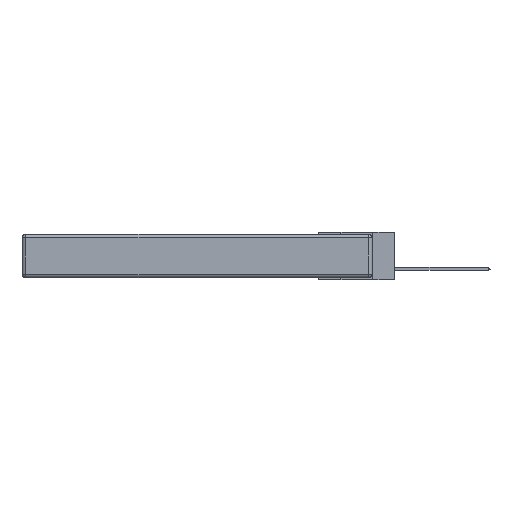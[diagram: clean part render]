
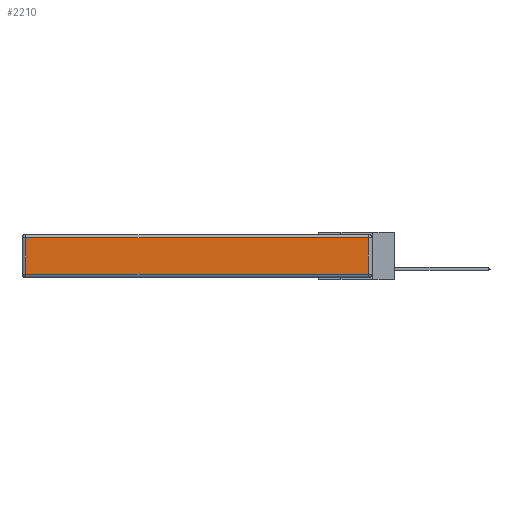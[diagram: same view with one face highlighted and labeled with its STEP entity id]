
A CAD part, left-side view. The second image highlights one B-rep face of the part: STEP entity #2210.
In plain terms, the highlighted planar face has unit normal (-1, 0, 0).
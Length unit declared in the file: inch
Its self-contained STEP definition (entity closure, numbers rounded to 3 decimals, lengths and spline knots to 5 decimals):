
#1325 = FACE_OUTER_BOUND ( 'NONE', #23199, .T. ) ;
#1782 = CARTESIAN_POINT ( 'NONE',  ( 0., 2.72, -0.343 ) ) ;
#2210 = ADVANCED_FACE ( 'NONE', ( #1325 ), #20587, .T. ) ;
#2214 = DIRECTION ( 'NONE',  ( 0., 0., 1. ) ) ;
#4475 = VECTOR ( 'NONE', #23477, 39.37008 ) ;
#6830 = CARTESIAN_POINT ( 'NONE',  ( 0., 0.03, -0.343 ) ) ;
#8288 = ORIENTED_EDGE ( 'NONE', *, *, #9230, .T. ) ;
#8354 = ORIENTED_EDGE ( 'NONE', *, *, #14554, .T. ) ;
#8678 = DIRECTION ( 'NONE',  ( 0., 0., 1. ) ) ;
#8729 = VECTOR ( 'NONE', #8678, 39.37008 ) ;
#9230 = EDGE_CURVE ( 'NONE', #17596, #16946, #21676, .T. ) ;
#9329 = LINE ( 'NONE', #11516, #4475 ) ;
#9456 = VERTEX_POINT ( 'NONE', #12620 ) ;
#10346 = DIRECTION ( 'NONE',  ( 0., 1., 0. ) ) ;
#10718 = EDGE_CURVE ( 'NONE', #9456, #15543, #23298, .T. ) ;
#11516 = CARTESIAN_POINT ( 'NONE',  ( 0., 0., -0.313 ) ) ;
#12620 = CARTESIAN_POINT ( 'NONE',  ( 0., 0.03, -0.313 ) ) ;
#12637 = CARTESIAN_POINT ( 'NONE',  ( 0., 0.03, -0.03 ) ) ;
#13146 = DIRECTION ( 'NONE',  ( -1., 0., 0. ) ) ;
#14554 = EDGE_CURVE ( 'NONE', #15543, #17596, #21529, .T. ) ;
#14669 = VECTOR ( 'NONE', #10346, 39.37008 ) ;
#14853 = EDGE_CURVE ( 'NONE', #16946, #9456, #9329, .T. ) ;
#14921 = CARTESIAN_POINT ( 'NONE',  ( 0., 0., -0.343 ) ) ;
#15543 = VERTEX_POINT ( 'NONE', #12637 ) ;
#16946 = VERTEX_POINT ( 'NONE', #19606 ) ;
#17596 = VERTEX_POINT ( 'NONE', #22186 ) ;
#18137 = ORIENTED_EDGE ( 'NONE', *, *, #10718, .T. ) ;
#18841 = AXIS2_PLACEMENT_3D ( 'NONE', #14921, #13146, #2214 ) ;
#19606 = CARTESIAN_POINT ( 'NONE',  ( 0., 2.72, -0.313 ) ) ;
#19673 = VECTOR ( 'NONE', #21912, 39.37008 ) ;
#19680 = CARTESIAN_POINT ( 'NONE',  ( 0., 2.75, -0.03 ) ) ;
#20587 = PLANE ( 'NONE',  #18841 ) ;
#21529 = LINE ( 'NONE', #19680, #14669 ) ;
#21561 = ORIENTED_EDGE ( 'NONE', *, *, #14853, .T. ) ;
#21676 = LINE ( 'NONE', #1782, #19673 ) ;
#21912 = DIRECTION ( 'NONE',  ( 0., 0., -1. ) ) ;
#22186 = CARTESIAN_POINT ( 'NONE',  ( 0., 2.72, -0.03 ) ) ;
#23199 = EDGE_LOOP ( 'NONE', ( #21561, #18137, #8354, #8288 ) ) ;
#23298 = LINE ( 'NONE', #6830, #8729 ) ;
#23477 = DIRECTION ( 'NONE',  ( 0., -1., 0. ) ) ;
